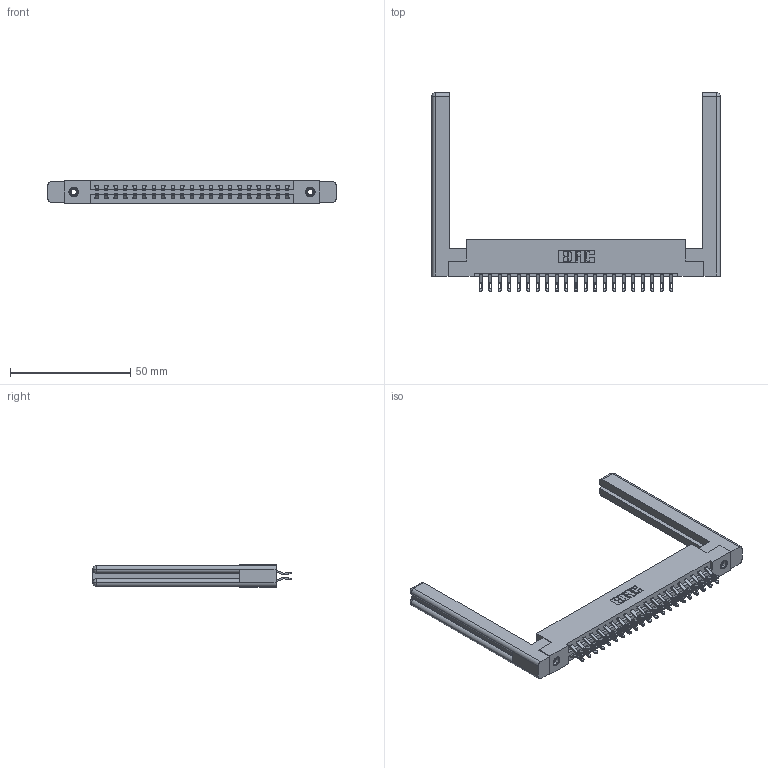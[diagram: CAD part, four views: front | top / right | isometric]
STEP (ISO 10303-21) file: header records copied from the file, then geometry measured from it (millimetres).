
FILE_DESCRIPTION (( 'STEP AP203' ), '1' );
FILE_NAME ('337-042-555-258.STEP', '2019-10-09T12:28:33', ( '' ), ( '' ), 'SwSTEP 2.0', 'SolidWorks 2016', '' );
FILE_SCHEMA (( 'CONFIG_CONTROL_DESIGN' ));
Length unit declared in the file: inch
Products named in the file (5): 337 Part_Flush Mounting Lugs - 0.156 Dia-TI; 345-250-001_345-250-001-102; 337-042-555-258; 345-292-001_555 Tail; 307-220-058
Assembly tree (47 placements, depth 2):
  337-042-555-258
    337 Part_Flush Mounting Lugs - 0.156 Dia-TI
    345-292-001_555 Tail  x42
    345-250-001_345-250-001-102  x2
    307-220-058  x2
Bounding box: 119.84 x 82.56 x 9.4 mm (x, y, z)
Volume: 19614 mm3; surface area: 19401.1 mm2
Topology: 47 solids, 47 shells, 2776 faces, 8603 edges, 5722 vertices
Faces by surface type: plane 1666, cylinder 1086, cone 12, torus 12
Entity records: 21958 total; most frequent: CARTESIAN_POINT 3759, ORIENTED_EDGE 3604, DIRECTION 3222, EDGE_CURVE 1802, LINE 1606, VECTOR 1606, VERTEX_POINT 1194, AXIS2_PLACEMENT_3D 808
